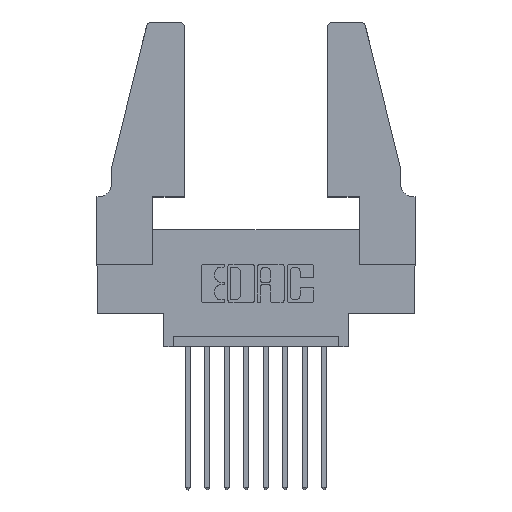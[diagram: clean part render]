
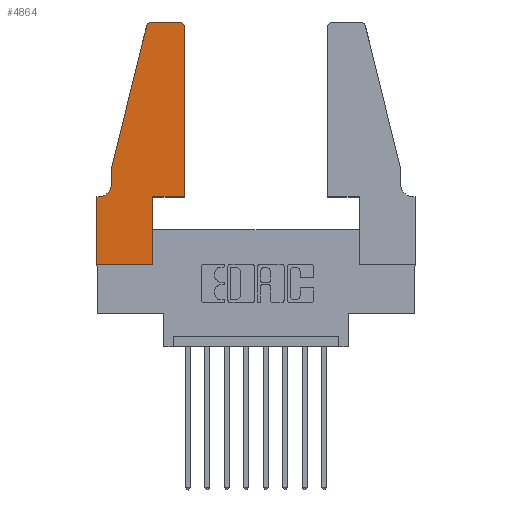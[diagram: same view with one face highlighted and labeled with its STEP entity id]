
A CAD part, top view. The second image highlights one B-rep face of the part: STEP entity #4864.
In plain terms, the highlighted planar face has unit normal (0, 0, 1).
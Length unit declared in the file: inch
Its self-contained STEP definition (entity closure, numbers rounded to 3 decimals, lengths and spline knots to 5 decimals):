
#125 = AXIS2_PLACEMENT_3D ( 'NONE', #11472, #12528, #11566 ) ;
#439 = LINE ( 'NONE', #2035, #9174 ) ;
#548 = CARTESIAN_POINT ( 'NONE',  ( 0., 0., 0.37 ) ) ;
#564 = ORIENTED_EDGE ( 'NONE', *, *, #2045, .T. ) ;
#823 = VERTEX_POINT ( 'NONE', #7616 ) ;
#903 = VERTEX_POINT ( 'NONE', #3191 ) ;
#915 = FACE_OUTER_BOUND ( 'NONE', #3082, .T. ) ;
#1001 = VERTEX_POINT ( 'NONE', #6133 ) ;
#1387 = VECTOR ( 'NONE', #7198, 39.37008 ) ;
#1470 = EDGE_CURVE ( 'NONE', #9344, #6293, #10046, .T. ) ;
#1546 = ORIENTED_EDGE ( 'NONE', *, *, #8220, .T. ) ;
#1659 = PLANE ( 'NONE',  #2316 ) ;
#1719 = CARTESIAN_POINT ( 'NONE',  ( 0.0755, 0.5, 0.37 ) ) ;
#1916 = ORIENTED_EDGE ( 'NONE', *, *, #11088, .T. ) ;
#2003 = ORIENTED_EDGE ( 'NONE', *, *, #1470, .T. ) ;
#2035 = CARTESIAN_POINT ( 'NONE',  ( 0., 0., 0.37 ) ) ;
#2036 = ORIENTED_EDGE ( 'NONE', *, *, #4812, .T. ) ;
#2045 = EDGE_CURVE ( 'NONE', #9409, #4108, #5198, .T. ) ;
#2184 = EDGE_CURVE ( 'NONE', #11286, #9474, #10468, .T. ) ;
#2237 = VECTOR ( 'NONE', #6584, 39.37008 ) ;
#2316 = AXIS2_PLACEMENT_3D ( 'NONE', #8573, #3697, #11500 ) ;
#2345 = CARTESIAN_POINT ( 'NONE',  ( 0.2865, 0.35, 0.37 ) ) ;
#2447 = AXIS2_PLACEMENT_3D ( 'NONE', #12168, #4190, #11138 ) ;
#2762 = CARTESIAN_POINT ( 'NONE',  ( 0.4505, 0.35, 0.37 ) ) ;
#3082 = EDGE_LOOP ( 'NONE', ( #3797, #9811, #8570, #1916, #11020, #9109, #564, #5411, #1546, #10993, #2036, #2003 ) ) ;
#3191 = CARTESIAN_POINT ( 'NONE',  ( 0.0755, 0.42, 0.37 ) ) ;
#3413 = DIRECTION ( 'NONE',  ( -1., 0., 0. ) ) ;
#3697 = DIRECTION ( 'NONE',  ( 0., 0., 1. ) ) ;
#3757 = EDGE_CURVE ( 'NONE', #823, #1001, #11862, .T. ) ;
#3797 = ORIENTED_EDGE ( 'NONE', *, *, #10363, .T. ) ;
#4021 = LINE ( 'NONE', #2345, #1387 ) ;
#4035 = VECTOR ( 'NONE', #10774, 39.37008 ) ;
#4049 = DIRECTION ( 'NONE',  ( -1., 0., 0. ) ) ;
#4092 = CARTESIAN_POINT ( 'NONE',  ( 0.2605, 1.25, 0.37 ) ) ;
#4108 = VERTEX_POINT ( 'NONE', #7281 ) ;
#4190 = DIRECTION ( 'NONE',  ( 0., 0., 1. ) ) ;
#4290 = LINE ( 'NONE', #4092, #4596 ) ;
#4337 = VERTEX_POINT ( 'NONE', #1719 ) ;
#4420 = DIRECTION ( 'NONE',  ( -1., 0., 0. ) ) ;
#4492 = CARTESIAN_POINT ( 'NONE',  ( 0.0055, 0.35, 0.37 ) ) ;
#4596 = VECTOR ( 'NONE', #4049, 39.37008 ) ;
#4678 = CARTESIAN_POINT ( 'NONE',  ( 0.4505, 0.35, 0.37 ) ) ;
#4812 = EDGE_CURVE ( 'NONE', #9474, #9344, #11994, .T. ) ;
#4864 = ADVANCED_FACE ( 'NONE', ( #915 ), #1659, .T. ) ;
#5198 = LINE ( 'NONE', #548, #5497 ) ;
#5411 = ORIENTED_EDGE ( 'NONE', *, *, #8090, .T. ) ;
#5497 = VECTOR ( 'NONE', #11755, 39.37008 ) ;
#5821 = CARTESIAN_POINT ( 'NONE',  ( 0.4505, 0.35, 0.37 ) ) ;
#6133 = CARTESIAN_POINT ( 'NONE',  ( 0.25487, 1.22718, 0.37 ) ) ;
#6281 = CARTESIAN_POINT ( 'NONE',  ( 0.0055, 0.42, 0.37 ) ) ;
#6293 = VERTEX_POINT ( 'NONE', #11074 ) ;
#6584 = DIRECTION ( 'NONE',  ( 1., 0., 0. ) ) ;
#6667 = VECTOR ( 'NONE', #10467, 39.37008 ) ;
#6810 = CARTESIAN_POINT ( 'NONE',  ( 0.0755, 0.5, 0.37 ) ) ;
#6920 = CARTESIAN_POINT ( 'NONE',  ( 0.4505, 1.22, 0.37 ) ) ;
#7198 = DIRECTION ( 'NONE',  ( 0., 1., 0. ) ) ;
#7281 = CARTESIAN_POINT ( 'NONE',  ( 0., 0., 0.37 ) ) ;
#7616 = CARTESIAN_POINT ( 'NONE',  ( 0.284, 1.25, 0.37 ) ) ;
#7947 = EDGE_CURVE ( 'NONE', #1001, #4337, #8861, .T. ) ;
#8090 = EDGE_CURVE ( 'NONE', #4108, #11007, #439, .T. ) ;
#8220 = EDGE_CURVE ( 'NONE', #11007, #11286, #4021, .T. ) ;
#8570 = ORIENTED_EDGE ( 'NONE', *, *, #7947, .T. ) ;
#8573 = CARTESIAN_POINT ( 'NONE',  ( 0., 0.35, 0.37 ) ) ;
#8656 = EDGE_CURVE ( 'NONE', #9360, #9409, #11327, .T. ) ;
#8861 = LINE ( 'NONE', #6810, #4035 ) ;
#8913 = CARTESIAN_POINT ( 'NONE',  ( 0., 0.35, 0.37 ) ) ;
#9002 = DIRECTION ( 'NONE',  ( 1., 0., 0. ) ) ;
#9085 = LINE ( 'NONE', #9970, #9252 ) ;
#9109 = ORIENTED_EDGE ( 'NONE', *, *, #8656, .T. ) ;
#9174 = VECTOR ( 'NONE', #9002, 39.37008 ) ;
#9252 = VECTOR ( 'NONE', #11989, 39.37008 ) ;
#9344 = VERTEX_POINT ( 'NONE', #6920 ) ;
#9360 = VERTEX_POINT ( 'NONE', #4492 ) ;
#9366 = CARTESIAN_POINT ( 'NONE',  ( 0.2865, 0., 0.37 ) ) ;
#9409 = VERTEX_POINT ( 'NONE', #8913 ) ;
#9474 = VERTEX_POINT ( 'NONE', #5821 ) ;
#9811 = ORIENTED_EDGE ( 'NONE', *, *, #3757, .T. ) ;
#9970 = CARTESIAN_POINT ( 'NONE',  ( 0.0755, 0.5, 0.37 ) ) ;
#10037 = EDGE_CURVE ( 'NONE', #903, #9360, #11947, .T. ) ;
#10046 = CIRCLE ( 'NONE', #2447, 0.03 ) ;
#10250 = VECTOR ( 'NONE', #3413, 39.37008 ) ;
#10363 = EDGE_CURVE ( 'NONE', #6293, #823, #4290, .T. ) ;
#10467 = DIRECTION ( 'NONE',  ( 0., 1., 0. ) ) ;
#10468 = LINE ( 'NONE', #2762, #2237 ) ;
#10774 = DIRECTION ( 'NONE',  ( -0.239, -0.971, 0. ) ) ;
#10993 = ORIENTED_EDGE ( 'NONE', *, *, #2184, .T. ) ;
#11007 = VERTEX_POINT ( 'NONE', #9366 ) ;
#11020 = ORIENTED_EDGE ( 'NONE', *, *, #10037, .T. ) ;
#11074 = CARTESIAN_POINT ( 'NONE',  ( 0.4205, 1.25, 0.37 ) ) ;
#11088 = EDGE_CURVE ( 'NONE', #4337, #903, #9085, .T. ) ;
#11138 = DIRECTION ( 'NONE',  ( 1., 0., 0. ) ) ;
#11265 = CARTESIAN_POINT ( 'NONE',  ( 0.2865, 0.35, 0.37 ) ) ;
#11286 = VERTEX_POINT ( 'NONE', #11265 ) ;
#11293 = CARTESIAN_POINT ( 'NONE',  ( 0.0755, 0.35, 0.37 ) ) ;
#11327 = LINE ( 'NONE', #11293, #10250 ) ;
#11472 = CARTESIAN_POINT ( 'NONE',  ( 0.284, 1.22, 0.37 ) ) ;
#11500 = DIRECTION ( 'NONE',  ( 1., 0., 0. ) ) ;
#11566 = DIRECTION ( 'NONE',  ( 1., 0., 0. ) ) ;
#11755 = DIRECTION ( 'NONE',  ( 0., -1., 0. ) ) ;
#11862 = CIRCLE ( 'NONE', #125, 0.03 ) ;
#11947 = CIRCLE ( 'NONE', #12787, 0.07 ) ;
#11989 = DIRECTION ( 'NONE',  ( 0., -1., 0. ) ) ;
#11994 = LINE ( 'NONE', #4678, #6667 ) ;
#12168 = CARTESIAN_POINT ( 'NONE',  ( 0.4205, 1.22, 0.37 ) ) ;
#12310 = DIRECTION ( 'NONE',  ( 0., 0., -1. ) ) ;
#12528 = DIRECTION ( 'NONE',  ( 0., 0., 1. ) ) ;
#12787 = AXIS2_PLACEMENT_3D ( 'NONE', #6281, #12310, #4420 ) ;
